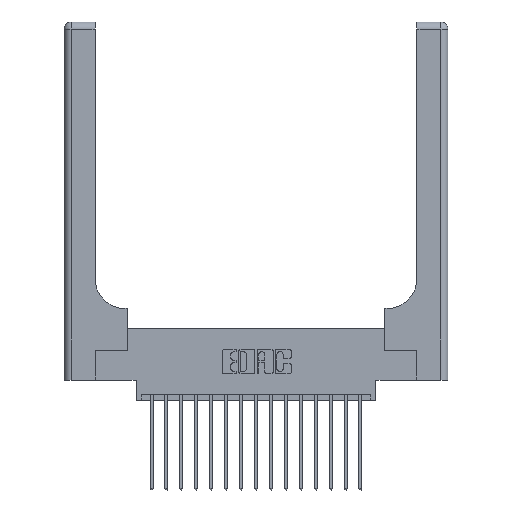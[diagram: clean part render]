
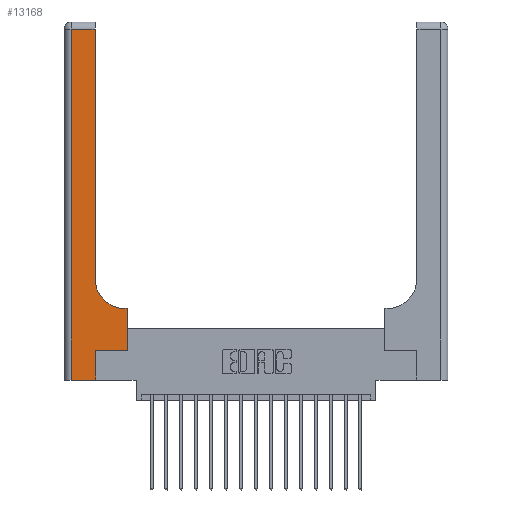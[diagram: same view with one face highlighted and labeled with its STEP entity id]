
A CAD part, top view. The second image highlights one B-rep face of the part: STEP entity #13168.
In plain terms, the highlighted planar face has unit normal (0, 0, 1).
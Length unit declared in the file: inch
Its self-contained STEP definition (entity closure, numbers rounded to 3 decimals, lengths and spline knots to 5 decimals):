
#323 = DIRECTION ( 'NONE',  ( -1., 0., 0. ) ) ;
#439 = VERTEX_POINT ( 'NONE', #16459 ) ;
#630 = VECTOR ( 'NONE', #12751, 39.37008 ) ;
#697 = EDGE_LOOP ( 'NONE', ( #13550, #18831, #15964, #13851, #1912, #12059, #4341, #15284, #2367 ) ) ;
#1278 = VERTEX_POINT ( 'NONE', #17454 ) ;
#1695 = CARTESIAN_POINT ( 'NONE',  ( 0.06, 0., 0.37 ) ) ;
#1912 = ORIENTED_EDGE ( 'NONE', *, *, #12298, .T. ) ;
#1917 = VERTEX_POINT ( 'NONE', #7881 ) ;
#2367 = ORIENTED_EDGE ( 'NONE', *, *, #15255, .T. ) ;
#2472 = VERTEX_POINT ( 'NONE', #6772 ) ;
#3190 = CARTESIAN_POINT ( 'NONE',  ( 0.528, 0.25, 0.37 ) ) ;
#3322 = VERTEX_POINT ( 'NONE', #14043 ) ;
#3573 = FACE_OUTER_BOUND ( 'NONE', #697, .T. ) ;
#4140 = CARTESIAN_POINT ( 'NONE',  ( 0.26, 3., 0.37 ) ) ;
#4216 = CARTESIAN_POINT ( 'NONE',  ( 0.06, 2.94, 0.37 ) ) ;
#4341 = ORIENTED_EDGE ( 'NONE', *, *, #9350, .T. ) ;
#4560 = AXIS2_PLACEMENT_3D ( 'NONE', #12099, #4708, #18971 ) ;
#4708 = DIRECTION ( 'NONE',  ( 0., 0., -1. ) ) ;
#6114 = CIRCLE ( 'NONE', #4560, 0.25 ) ;
#6772 = CARTESIAN_POINT ( 'NONE',  ( 0.265, 0., 0.37 ) ) ;
#6809 = VECTOR ( 'NONE', #14515, 39.37008 ) ;
#7565 = CARTESIAN_POINT ( 'NONE',  ( 0.265, 0., 0.37 ) ) ;
#7646 = VECTOR ( 'NONE', #323, 39.37008 ) ;
#7881 = CARTESIAN_POINT ( 'NONE',  ( 0.265, 0.25, 0.37 ) ) ;
#8351 = LINE ( 'NONE', #16098, #16055 ) ;
#8634 = DIRECTION ( 'NONE',  ( -1., 0., 0. ) ) ;
#9040 = LINE ( 'NONE', #7565, #10289 ) ;
#9057 = EDGE_CURVE ( 'NONE', #439, #11484, #10708, .T. ) ;
#9350 = EDGE_CURVE ( 'NONE', #17793, #17761, #17312, .T. ) ;
#10234 = LINE ( 'NONE', #19167, #6809 ) ;
#10289 = VECTOR ( 'NONE', #18063, 39.37008 ) ;
#10708 = LINE ( 'NONE', #16623, #7646 ) ;
#11341 = LINE ( 'NONE', #19022, #12619 ) ;
#11484 = VERTEX_POINT ( 'NONE', #4216 ) ;
#11546 = LINE ( 'NONE', #4140, #12015 ) ;
#11969 = EDGE_CURVE ( 'NONE', #16995, #2472, #10234, .T. ) ;
#12015 = VECTOR ( 'NONE', #17556, 39.37008 ) ;
#12059 = ORIENTED_EDGE ( 'NONE', *, *, #18016, .T. ) ;
#12099 = CARTESIAN_POINT ( 'NONE',  ( 0.51, 0.85, 0.37 ) ) ;
#12298 = EDGE_CURVE ( 'NONE', #2472, #1917, #9040, .T. ) ;
#12619 = VECTOR ( 'NONE', #8634, 39.37008 ) ;
#12751 = DIRECTION ( 'NONE',  ( 0., 1., 0. ) ) ;
#13168 = ADVANCED_FACE ( 'NONE', ( #3573 ), #18736, .F. ) ;
#13550 = ORIENTED_EDGE ( 'NONE', *, *, #16826, .T. ) ;
#13851 = ORIENTED_EDGE ( 'NONE', *, *, #11969, .T. ) ;
#14043 = CARTESIAN_POINT ( 'NONE',  ( 0.26, 0.85, 0.37 ) ) ;
#14140 = AXIS2_PLACEMENT_3D ( 'NONE', #15537, #15726, #17180 ) ;
#14439 = DIRECTION ( 'NONE',  ( 0., -1., 0. ) ) ;
#14515 = DIRECTION ( 'NONE',  ( 1., 0., 0. ) ) ;
#15255 = EDGE_CURVE ( 'NONE', #1278, #3322, #6114, .T. ) ;
#15284 = ORIENTED_EDGE ( 'NONE', *, *, #16853, .T. ) ;
#15537 = CARTESIAN_POINT ( 'NONE',  ( 0., 3., 0.37 ) ) ;
#15726 = DIRECTION ( 'NONE',  ( 0., 0., -1. ) ) ;
#15964 = ORIENTED_EDGE ( 'NONE', *, *, #18331, .T. ) ;
#16055 = VECTOR ( 'NONE', #17173, 39.37008 ) ;
#16098 = CARTESIAN_POINT ( 'NONE',  ( 0.265, 0.25, 0.37 ) ) ;
#16459 = CARTESIAN_POINT ( 'NONE',  ( 0.26, 2.94, 0.37 ) ) ;
#16623 = CARTESIAN_POINT ( 'NONE',  ( 0., 2.94, 0.37 ) ) ;
#16826 = EDGE_CURVE ( 'NONE', #3322, #439, #11546, .T. ) ;
#16853 = EDGE_CURVE ( 'NONE', #17761, #1278, #11341, .T. ) ;
#16995 = VERTEX_POINT ( 'NONE', #1695 ) ;
#17150 = CARTESIAN_POINT ( 'NONE',  ( 0.06, 3., 0.37 ) ) ;
#17173 = DIRECTION ( 'NONE',  ( 1., 0., 0. ) ) ;
#17180 = DIRECTION ( 'NONE',  ( -1., 0., 0. ) ) ;
#17312 = LINE ( 'NONE', #17411, #630 ) ;
#17411 = CARTESIAN_POINT ( 'NONE',  ( 0.528, 0.25, 0.37 ) ) ;
#17454 = CARTESIAN_POINT ( 'NONE',  ( 0.51, 0.6, 0.37 ) ) ;
#17534 = LINE ( 'NONE', #17150, #18236 ) ;
#17556 = DIRECTION ( 'NONE',  ( 0., 1., 0. ) ) ;
#17761 = VERTEX_POINT ( 'NONE', #17773 ) ;
#17773 = CARTESIAN_POINT ( 'NONE',  ( 0.528, 0.6, 0.37 ) ) ;
#17793 = VERTEX_POINT ( 'NONE', #3190 ) ;
#18016 = EDGE_CURVE ( 'NONE', #1917, #17793, #8351, .T. ) ;
#18063 = DIRECTION ( 'NONE',  ( 0., 1., 0. ) ) ;
#18236 = VECTOR ( 'NONE', #14439, 39.37008 ) ;
#18331 = EDGE_CURVE ( 'NONE', #11484, #16995, #17534, .T. ) ;
#18736 = PLANE ( 'NONE',  #14140 ) ;
#18831 = ORIENTED_EDGE ( 'NONE', *, *, #9057, .T. ) ;
#18971 = DIRECTION ( 'NONE',  ( 1., 0., 0. ) ) ;
#19022 = CARTESIAN_POINT ( 'NONE',  ( 0.26, 0.6, 0.37 ) ) ;
#19167 = CARTESIAN_POINT ( 'NONE',  ( 0., 0., 0.37 ) ) ;
